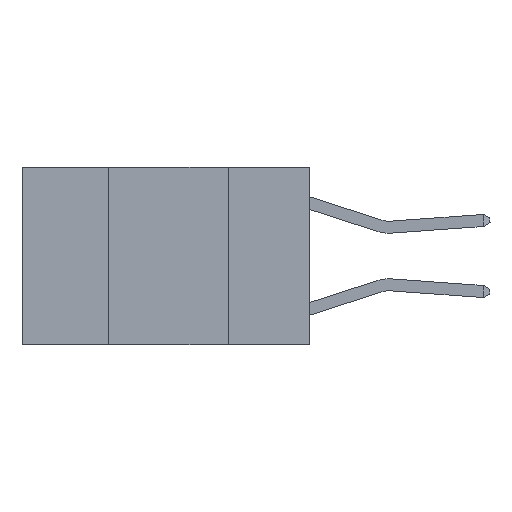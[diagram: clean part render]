
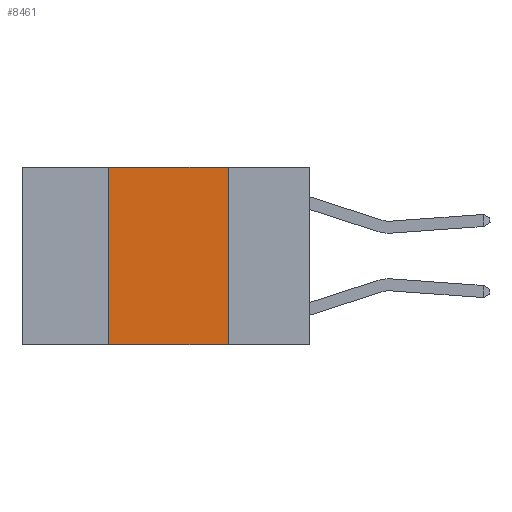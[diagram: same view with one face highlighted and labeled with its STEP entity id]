
A CAD part, left-side view. The second image highlights one B-rep face of the part: STEP entity #8461.
In plain terms, the highlighted planar face has unit normal (-1, 0, 0).
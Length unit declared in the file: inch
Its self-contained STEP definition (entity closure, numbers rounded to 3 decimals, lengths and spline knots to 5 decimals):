
#433 = FACE_OUTER_BOUND ( 'NONE', #8442, .T. ) ;
#2026 = PLANE ( 'NONE',  #13496 ) ;
#3042 = EDGE_CURVE ( 'NONE', #5287, #12988, #6843, .T. ) ;
#3087 = CARTESIAN_POINT ( 'NONE',  ( 0., 0.42, 0. ) ) ;
#3122 = ORIENTED_EDGE ( 'NONE', *, *, #9814, .F. ) ;
#3150 = DIRECTION ( 'NONE',  ( 0., 0., -1. ) ) ;
#3161 = CARTESIAN_POINT ( 'NONE',  ( 0., 0.6, 0. ) ) ;
#3666 = CARTESIAN_POINT ( 'NONE',  ( 0., 0.17, 0. ) ) ;
#3891 = CARTESIAN_POINT ( 'NONE',  ( 0., 0.17, -0.37 ) ) ;
#3906 = EDGE_CURVE ( 'NONE', #5287, #7657, #11712, .T. ) ;
#4198 = ORIENTED_EDGE ( 'NONE', *, *, #3042, .T. ) ;
#4320 = DIRECTION ( 'NONE',  ( 0., -1., 0. ) ) ;
#5287 = VERTEX_POINT ( 'NONE', #12206 ) ;
#5386 = DIRECTION ( 'NONE',  ( 0., 0., 1. ) ) ;
#5821 = VECTOR ( 'NONE', #4320, 39.37008 ) ;
#6181 = ORIENTED_EDGE ( 'NONE', *, *, #10607, .F. ) ;
#6207 = LINE ( 'NONE', #3161, #5821 ) ;
#6428 = VECTOR ( 'NONE', #14352, 39.37008 ) ;
#6843 = LINE ( 'NONE', #12719, #7204 ) ;
#7204 = VECTOR ( 'NONE', #10897, 39.37008 ) ;
#7485 = CARTESIAN_POINT ( 'NONE',  ( 0., 0.42, 0. ) ) ;
#7553 = CARTESIAN_POINT ( 'NONE',  ( 0., 0.17, 0. ) ) ;
#7657 = VERTEX_POINT ( 'NONE', #7485 ) ;
#8442 = EDGE_LOOP ( 'NONE', ( #3122, #6181, #12560, #4198 ) ) ;
#8461 = ADVANCED_FACE ( 'NONE', ( #433 ), #2026, .F. ) ;
#8714 = VECTOR ( 'NONE', #5386, 39.37008 ) ;
#9445 = LINE ( 'NONE', #7553, #6428 ) ;
#9814 = EDGE_CURVE ( 'NONE', #10244, #12988, #9445, .T. ) ;
#9985 = DIRECTION ( 'NONE',  ( 1., 0., 0. ) ) ;
#10244 = VERTEX_POINT ( 'NONE', #3666 ) ;
#10607 = EDGE_CURVE ( 'NONE', #7657, #10244, #6207, .T. ) ;
#10897 = DIRECTION ( 'NONE',  ( 0., -1., 0. ) ) ;
#11041 = CARTESIAN_POINT ( 'NONE',  ( 0., 0.6, 0. ) ) ;
#11712 = LINE ( 'NONE', #3087, #8714 ) ;
#12206 = CARTESIAN_POINT ( 'NONE',  ( 0., 0.42, -0.37 ) ) ;
#12560 = ORIENTED_EDGE ( 'NONE', *, *, #3906, .F. ) ;
#12719 = CARTESIAN_POINT ( 'NONE',  ( 0., 0.6, -0.37 ) ) ;
#12988 = VERTEX_POINT ( 'NONE', #3891 ) ;
#13496 = AXIS2_PLACEMENT_3D ( 'NONE', #11041, #9985, #3150 ) ;
#14352 = DIRECTION ( 'NONE',  ( 0., 0., -1. ) ) ;
